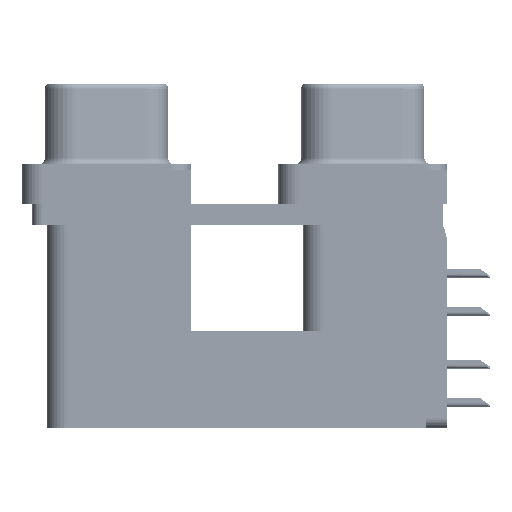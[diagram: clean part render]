
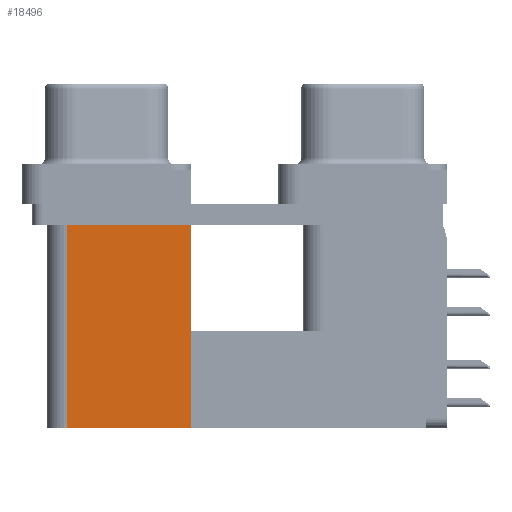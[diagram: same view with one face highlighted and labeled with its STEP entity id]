
A CAD part, left-side view. The second image highlights one B-rep face of the part: STEP entity #18496.
In plain terms, the highlighted planar face has unit normal (-1, 0, 0).
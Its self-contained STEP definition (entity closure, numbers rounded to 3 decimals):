
#1026 = VECTOR ( 'NONE', #24060, 1000. ) ;
#1056 = EDGE_CURVE ( 'NONE', #36598, #33252, #47419, .T. ) ;
#3191 = EDGE_LOOP ( 'NONE', ( #34529, #33482, #4705, #37419 ) ) ;
#3439 = EDGE_CURVE ( 'NONE', #41676, #37561, #39068, .T. ) ;
#4705 = ORIENTED_EDGE ( 'NONE', *, *, #29966, .F. ) ;
#7981 = LINE ( 'NONE', #36284, #27924 ) ;
#8370 = CARTESIAN_POINT ( 'NONE',  ( 3.79, 21.975, -19.2 ) ) ;
#16098 = VECTOR ( 'NONE', #22488, 1000. ) ;
#18496 = ADVANCED_FACE ( 'NONE', ( #37869 ), #29904, .F. ) ;
#19767 = CARTESIAN_POINT ( 'NONE',  ( 3.79, 12.775, -19.2 ) ) ;
#20434 = CARTESIAN_POINT ( 'NONE',  ( 3.79, 12.775, -19.2 ) ) ;
#21431 = AXIS2_PLACEMENT_3D ( 'NONE', #26559, #42219, #45813 ) ;
#22488 = DIRECTION ( 'NONE',  ( 0., 1., 0. ) ) ;
#23828 = VECTOR ( 'NONE', #27262, 1000. ) ;
#24060 = DIRECTION ( 'NONE',  ( 0., 0., 1. ) ) ;
#26559 = CARTESIAN_POINT ( 'NONE',  ( 3.79, 12.775, -19.2 ) ) ;
#27262 = DIRECTION ( 'NONE',  ( 0., 0., 1. ) ) ;
#27924 = VECTOR ( 'NONE', #47810, 1000. ) ;
#29904 = PLANE ( 'NONE',  #21431 ) ;
#29966 = EDGE_CURVE ( 'NONE', #41676, #36598, #50474, .T. ) ;
#31294 = CARTESIAN_POINT ( 'NONE',  ( 3.79, 21.975, -2.5 ) ) ;
#31962 = CARTESIAN_POINT ( 'NONE',  ( 3.79, 12.775, -2.5 ) ) ;
#33252 = VERTEX_POINT ( 'NONE', #31294 ) ;
#33482 = ORIENTED_EDGE ( 'NONE', *, *, #1056, .F. ) ;
#34529 = ORIENTED_EDGE ( 'NONE', *, *, #42546, .T. ) ;
#36284 = CARTESIAN_POINT ( 'NONE',  ( 3.79, 12.775, -2.5 ) ) ;
#36598 = VERTEX_POINT ( 'NONE', #40573 ) ;
#37419 = ORIENTED_EDGE ( 'NONE', *, *, #3439, .T. ) ;
#37561 = VERTEX_POINT ( 'NONE', #31962 ) ;
#37869 = FACE_OUTER_BOUND ( 'NONE', #3191, .T. ) ;
#39068 = LINE ( 'NONE', #19767, #23828 ) ;
#40573 = CARTESIAN_POINT ( 'NONE',  ( 3.79, 21.975, -19.2 ) ) ;
#41676 = VERTEX_POINT ( 'NONE', #20434 ) ;
#42219 = DIRECTION ( 'NONE',  ( 1., 0., 0. ) ) ;
#42546 = EDGE_CURVE ( 'NONE', #37561, #33252, #7981, .T. ) ;
#45813 = DIRECTION ( 'NONE',  ( 0., 0., -1. ) ) ;
#47419 = LINE ( 'NONE', #8370, #1026 ) ;
#47810 = DIRECTION ( 'NONE',  ( 0., 1., 0. ) ) ;
#50232 = CARTESIAN_POINT ( 'NONE',  ( 3.79, 12.775, -19.2 ) ) ;
#50474 = LINE ( 'NONE', #50232, #16098 ) ;
